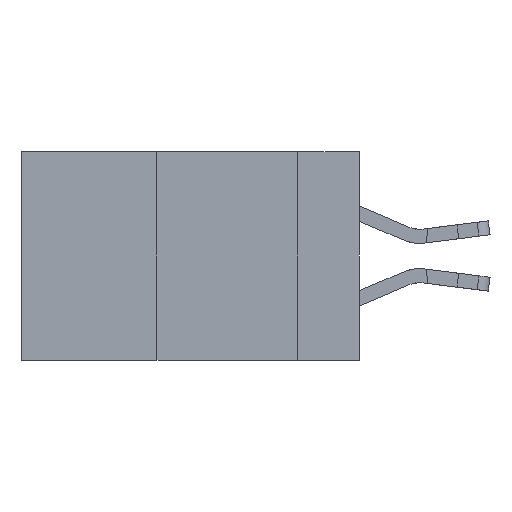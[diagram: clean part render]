
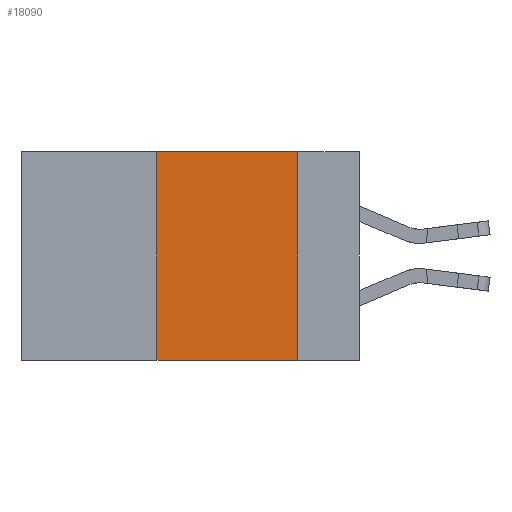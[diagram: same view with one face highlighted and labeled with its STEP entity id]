
A CAD part, left-side view. The second image highlights one B-rep face of the part: STEP entity #18090.
In plain terms, the highlighted planar face has unit normal (-1, 0, 0).
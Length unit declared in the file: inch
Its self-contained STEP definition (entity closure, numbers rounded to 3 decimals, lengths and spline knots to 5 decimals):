
#277 = ORIENTED_EDGE ( 'NONE', *, *, #4711, .F. ) ;
#1461 = LINE ( 'NONE', #21607, #22886 ) ;
#1807 = VERTEX_POINT ( 'NONE', #21102 ) ;
#2556 = ORIENTED_EDGE ( 'NONE', *, *, #19184, .F. ) ;
#2742 = CARTESIAN_POINT ( 'NONE',  ( 0., 0.11, 0. ) ) ;
#4617 = PLANE ( 'NONE',  #24761 ) ;
#4711 = EDGE_CURVE ( 'NONE', #20134, #1807, #1461, .T. ) ;
#4788 = CARTESIAN_POINT ( 'NONE',  ( 0., 0.6, 0. ) ) ;
#4886 = DIRECTION ( 'NONE',  ( 0., 0., 1. ) ) ;
#5544 = VERTEX_POINT ( 'NONE', #8385 ) ;
#6141 = CARTESIAN_POINT ( 'NONE',  ( 0., 0.6, 0. ) ) ;
#6358 = FACE_OUTER_BOUND ( 'NONE', #7978, .T. ) ;
#6747 = VERTEX_POINT ( 'NONE', #22600 ) ;
#7978 = EDGE_LOOP ( 'NONE', ( #277, #2556, #14517, #10045 ) ) ;
#8385 = CARTESIAN_POINT ( 'NONE',  ( 0., 0.36, 0. ) ) ;
#10045 = ORIENTED_EDGE ( 'NONE', *, *, #24623, .T. ) ;
#10477 = DIRECTION ( 'NONE',  ( 0., 0., -1. ) ) ;
#11020 = EDGE_CURVE ( 'NONE', #6747, #5544, #21831, .T. ) ;
#14517 = ORIENTED_EDGE ( 'NONE', *, *, #11020, .F. ) ;
#15625 = DIRECTION ( 'NONE',  ( 0., -1., 0. ) ) ;
#16296 = VECTOR ( 'NONE', #21053, 39.37008 ) ;
#17475 = DIRECTION ( 'NONE',  ( 0., 0., -1. ) ) ;
#18090 = ADVANCED_FACE ( 'NONE', ( #6358 ), #4617, .F. ) ;
#18212 = DIRECTION ( 'NONE',  ( 1., 0., 0. ) ) ;
#18993 = LINE ( 'NONE', #6141, #22294 ) ;
#19184 = EDGE_CURVE ( 'NONE', #5544, #20134, #18993, .T. ) ;
#20134 = VERTEX_POINT ( 'NONE', #2742 ) ;
#20238 = CARTESIAN_POINT ( 'NONE',  ( 0., 0.36, 0. ) ) ;
#21053 = DIRECTION ( 'NONE',  ( 0., -1., 0. ) ) ;
#21102 = CARTESIAN_POINT ( 'NONE',  ( 0., 0.11, -0.37 ) ) ;
#21150 = LINE ( 'NONE', #22891, #16296 ) ;
#21498 = VECTOR ( 'NONE', #4886, 39.37008 ) ;
#21607 = CARTESIAN_POINT ( 'NONE',  ( 0., 0.11, 0. ) ) ;
#21831 = LINE ( 'NONE', #20238, #21498 ) ;
#22294 = VECTOR ( 'NONE', #15625, 39.37008 ) ;
#22600 = CARTESIAN_POINT ( 'NONE',  ( 0., 0.36, -0.37 ) ) ;
#22886 = VECTOR ( 'NONE', #17475, 39.37008 ) ;
#22891 = CARTESIAN_POINT ( 'NONE',  ( 0., 0.6, -0.37 ) ) ;
#24623 = EDGE_CURVE ( 'NONE', #6747, #1807, #21150, .T. ) ;
#24761 = AXIS2_PLACEMENT_3D ( 'NONE', #4788, #18212, #10477 ) ;
